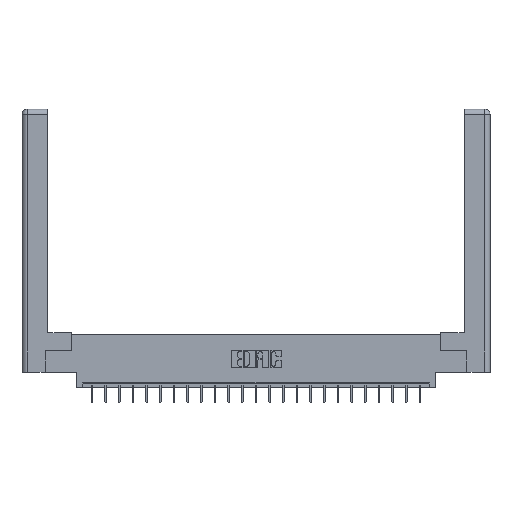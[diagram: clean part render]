
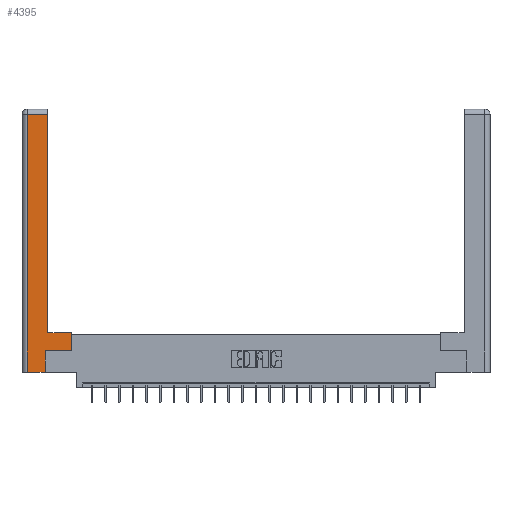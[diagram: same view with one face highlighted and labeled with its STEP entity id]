
A CAD part, top view. The second image highlights one B-rep face of the part: STEP entity #4395.
In plain terms, the highlighted planar face has unit normal (0, 0, 1).
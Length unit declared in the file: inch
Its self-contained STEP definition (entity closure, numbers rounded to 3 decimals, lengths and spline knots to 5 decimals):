
#159 = CARTESIAN_POINT ( 'NONE',  ( 0.295, 0.45, 0. ) ) ;
#693 = ORIENTED_EDGE ( 'NONE', *, *, #10153, .T. ) ;
#1037 = ORIENTED_EDGE ( 'NONE', *, *, #3794, .T. ) ;
#1313 = VECTOR ( 'NONE', #11748, 39.37008 ) ;
#1940 = CARTESIAN_POINT ( 'NONE',  ( 0.265, 0., 0. ) ) ;
#2235 = CARTESIAN_POINT ( 'NONE',  ( 0.295, 0.45, 0. ) ) ;
#2425 = LINE ( 'NONE', #4784, #6545 ) ;
#2807 = LINE ( 'NONE', #159, #1313 ) ;
#3050 = LINE ( 'NONE', #24203, #8072 ) ;
#3384 = EDGE_CURVE ( 'NONE', #8033, #21791, #3050, .T. ) ;
#3510 = DIRECTION ( 'NONE',  ( 0., 1., 0. ) ) ;
#3794 = EDGE_CURVE ( 'NONE', #21791, #17797, #6856, .T. ) ;
#3848 = DIRECTION ( 'NONE',  ( -1., 0., 0. ) ) ;
#3940 = ORIENTED_EDGE ( 'NONE', *, *, #14354, .T. ) ;
#4210 = CARTESIAN_POINT ( 'NONE',  ( 0.0615, 0., 0. ) ) ;
#4395 = ADVANCED_FACE ( 'NONE', ( #23341 ), #6490, .F. ) ;
#4784 = CARTESIAN_POINT ( 'NONE',  ( 0.565, 0.245, 0. ) ) ;
#4994 = VERTEX_POINT ( 'NONE', #20288 ) ;
#5464 = CARTESIAN_POINT ( 'NONE',  ( 0.265, 0., 0. ) ) ;
#6359 = EDGE_CURVE ( 'NONE', #8331, #8033, #19407, .T. ) ;
#6410 = DIRECTION ( 'NONE',  ( -1., 0., 0. ) ) ;
#6490 = PLANE ( 'NONE',  #8943 ) ;
#6545 = VECTOR ( 'NONE', #16541, 39.37008 ) ;
#6781 = DIRECTION ( 'NONE',  ( 0., 1., 0. ) ) ;
#6784 = EDGE_CURVE ( 'NONE', #17797, #22232, #7268, .T. ) ;
#6856 = LINE ( 'NONE', #5464, #20708 ) ;
#7268 = LINE ( 'NONE', #16113, #20253 ) ;
#7380 = DIRECTION ( 'NONE',  ( 0., -1., 0. ) ) ;
#7393 = CARTESIAN_POINT ( 'NONE',  ( 0.0615, 2.94, 0. ) ) ;
#8033 = VERTEX_POINT ( 'NONE', #7393 ) ;
#8072 = VECTOR ( 'NONE', #7380, 39.37008 ) ;
#8331 = VERTEX_POINT ( 'NONE', #21648 ) ;
#8943 = AXIS2_PLACEMENT_3D ( 'NONE', #16141, #18038, #6410 ) ;
#9694 = LINE ( 'NONE', #20757, #21185 ) ;
#9846 = LINE ( 'NONE', #22198, #18984 ) ;
#10153 = EDGE_CURVE ( 'NONE', #16697, #4994, #9694, .T. ) ;
#11748 = DIRECTION ( 'NONE',  ( -1., 0., 0. ) ) ;
#13486 = ORIENTED_EDGE ( 'NONE', *, *, #23843, .T. ) ;
#14354 = EDGE_CURVE ( 'NONE', #22232, #16697, #2425, .T. ) ;
#14974 = VECTOR ( 'NONE', #3848, 39.37008 ) ;
#16113 = CARTESIAN_POINT ( 'NONE',  ( 0.265, 0.245, 0. ) ) ;
#16141 = CARTESIAN_POINT ( 'NONE',  ( 0., 0., 0. ) ) ;
#16541 = DIRECTION ( 'NONE',  ( 1., 0., 0. ) ) ;
#16697 = VERTEX_POINT ( 'NONE', #20963 ) ;
#17797 = VERTEX_POINT ( 'NONE', #1940 ) ;
#18038 = DIRECTION ( 'NONE',  ( 0., 0., -1. ) ) ;
#18739 = DIRECTION ( 'NONE',  ( 1., 0., 0. ) ) ;
#18779 = DIRECTION ( 'NONE',  ( 0., 1., 0. ) ) ;
#18984 = VECTOR ( 'NONE', #3510, 39.37008 ) ;
#19362 = ORIENTED_EDGE ( 'NONE', *, *, #22402, .T. ) ;
#19407 = LINE ( 'NONE', #24447, #14974 ) ;
#20253 = VECTOR ( 'NONE', #6781, 39.37008 ) ;
#20288 = CARTESIAN_POINT ( 'NONE',  ( 0.565, 0.45, 0. ) ) ;
#20384 = ORIENTED_EDGE ( 'NONE', *, *, #6359, .T. ) ;
#20708 = VECTOR ( 'NONE', #18739, 39.37008 ) ;
#20757 = CARTESIAN_POINT ( 'NONE',  ( 0.565, 0.45, 0. ) ) ;
#20963 = CARTESIAN_POINT ( 'NONE',  ( 0.565, 0.245, 0. ) ) ;
#21185 = VECTOR ( 'NONE', #18779, 39.37008 ) ;
#21329 = VERTEX_POINT ( 'NONE', #2235 ) ;
#21648 = CARTESIAN_POINT ( 'NONE',  ( 0.295, 2.94, 0. ) ) ;
#21791 = VERTEX_POINT ( 'NONE', #4210 ) ;
#22117 = CARTESIAN_POINT ( 'NONE',  ( 0.265, 0.245, 0. ) ) ;
#22198 = CARTESIAN_POINT ( 'NONE',  ( 0.295, 3., 0. ) ) ;
#22232 = VERTEX_POINT ( 'NONE', #22117 ) ;
#22402 = EDGE_CURVE ( 'NONE', #4994, #21329, #2807, .T. ) ;
#22436 = ORIENTED_EDGE ( 'NONE', *, *, #6784, .T. ) ;
#22766 = ORIENTED_EDGE ( 'NONE', *, *, #3384, .T. ) ;
#23341 = FACE_OUTER_BOUND ( 'NONE', #23585, .T. ) ;
#23585 = EDGE_LOOP ( 'NONE', ( #13486, #20384, #22766, #1037, #22436, #3940, #693, #19362 ) ) ;
#23843 = EDGE_CURVE ( 'NONE', #21329, #8331, #9846, .T. ) ;
#24203 = CARTESIAN_POINT ( 'NONE',  ( 0.0615, 0., 0. ) ) ;
#24447 = CARTESIAN_POINT ( 'NONE',  ( 0.0615, 2.94, 0. ) ) ;
